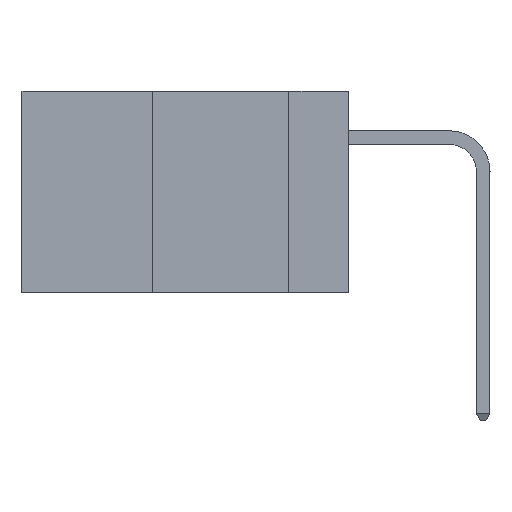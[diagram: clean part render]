
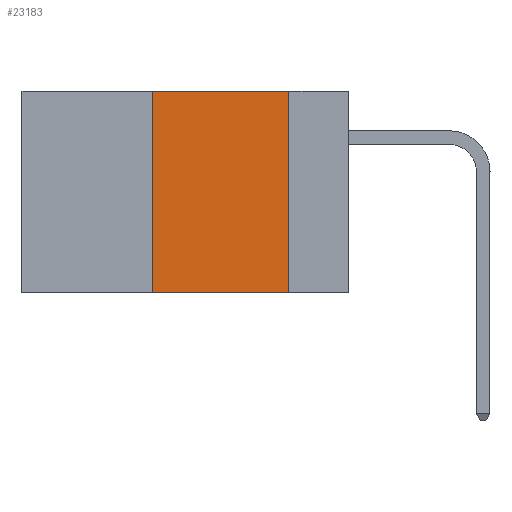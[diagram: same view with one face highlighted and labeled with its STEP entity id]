
A CAD part, left-side view. The second image highlights one B-rep face of the part: STEP entity #23183.
In plain terms, the highlighted planar face has unit normal (-1, 0, 0).
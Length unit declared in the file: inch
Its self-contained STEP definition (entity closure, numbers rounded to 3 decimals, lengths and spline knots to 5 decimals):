
#598 = CARTESIAN_POINT ( 'NONE',  ( 0., 0.11, -0.37 ) ) ;
#1767 = VECTOR ( 'NONE', #20398, 39.37008 ) ;
#1814 = DIRECTION ( 'NONE',  ( 0., 0., 1. ) ) ;
#2534 = LINE ( 'NONE', #7736, #35065 ) ;
#4148 = EDGE_CURVE ( 'NONE', #16245, #9039, #28989, .T. ) ;
#4223 = CARTESIAN_POINT ( 'NONE',  ( 0., 0.11, 0. ) ) ;
#7004 = ORIENTED_EDGE ( 'NONE', *, *, #4148, .F. ) ;
#7035 = LINE ( 'NONE', #12575, #15693 ) ;
#7736 = CARTESIAN_POINT ( 'NONE',  ( 0., 0.6, -0.37 ) ) ;
#9039 = VERTEX_POINT ( 'NONE', #16075 ) ;
#9373 = FACE_OUTER_BOUND ( 'NONE', #9437, .T. ) ;
#9433 = AXIS2_PLACEMENT_3D ( 'NONE', #14735, #19577, #20282 ) ;
#9437 = EDGE_LOOP ( 'NONE', ( #16939, #28640, #7004, #26012 ) ) ;
#12399 = DIRECTION ( 'NONE',  ( 0., -1., 0. ) ) ;
#12575 = CARTESIAN_POINT ( 'NONE',  ( 0., 0.6, 0. ) ) ;
#14153 = VECTOR ( 'NONE', #1814, 39.37008 ) ;
#14735 = CARTESIAN_POINT ( 'NONE',  ( 0., 0.6, 0. ) ) ;
#14843 = EDGE_CURVE ( 'NONE', #29300, #23153, #17172, .T. ) ;
#15693 = VECTOR ( 'NONE', #12399, 39.37008 ) ;
#16075 = CARTESIAN_POINT ( 'NONE',  ( 0., 0.36, 0. ) ) ;
#16245 = VERTEX_POINT ( 'NONE', #28262 ) ;
#16939 = ORIENTED_EDGE ( 'NONE', *, *, #14843, .F. ) ;
#17172 = LINE ( 'NONE', #28082, #1767 ) ;
#19577 = DIRECTION ( 'NONE',  ( 1., 0., 0. ) ) ;
#20282 = DIRECTION ( 'NONE',  ( 0., 0., -1. ) ) ;
#20398 = DIRECTION ( 'NONE',  ( 0., 0., -1. ) ) ;
#21140 = CARTESIAN_POINT ( 'NONE',  ( 0., 0.36, 0. ) ) ;
#23153 = VERTEX_POINT ( 'NONE', #598 ) ;
#23183 = ADVANCED_FACE ( 'NONE', ( #9373 ), #25473, .F. ) ;
#23259 = EDGE_CURVE ( 'NONE', #9039, #29300, #7035, .T. ) ;
#24358 = DIRECTION ( 'NONE',  ( 0., -1., 0. ) ) ;
#25473 = PLANE ( 'NONE',  #9433 ) ;
#26012 = ORIENTED_EDGE ( 'NONE', *, *, #32346, .T. ) ;
#28082 = CARTESIAN_POINT ( 'NONE',  ( 0., 0.11, 0. ) ) ;
#28262 = CARTESIAN_POINT ( 'NONE',  ( 0., 0.36, -0.37 ) ) ;
#28640 = ORIENTED_EDGE ( 'NONE', *, *, #23259, .F. ) ;
#28989 = LINE ( 'NONE', #21140, #14153 ) ;
#29300 = VERTEX_POINT ( 'NONE', #4223 ) ;
#32346 = EDGE_CURVE ( 'NONE', #16245, #23153, #2534, .T. ) ;
#35065 = VECTOR ( 'NONE', #24358, 39.37008 ) ;
